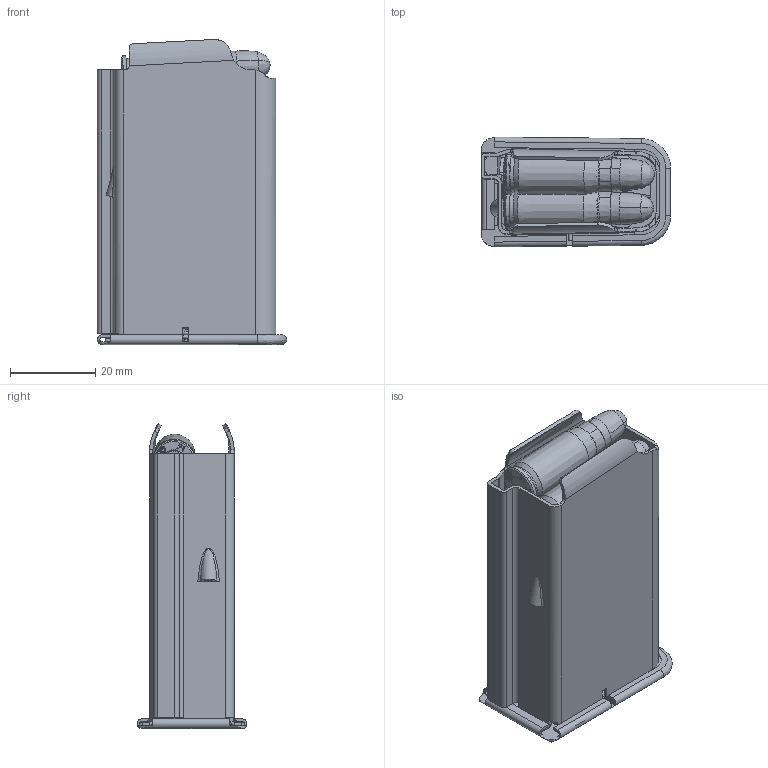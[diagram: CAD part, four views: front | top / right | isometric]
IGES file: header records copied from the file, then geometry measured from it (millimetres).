
Global section: file name: No Iges File Name specified; native system: Autodesk Inventor 2011; preprocessor: AutoDesk Inventor Iges Exporter R2011; author: EfimchenkoPA; date: 20111123.114528; units: millimetre
Bounding box: 44.5 x 25.86 x 71.75 mm (x, y, z)
Volume: 15185.1 mm3; surface area: 33232.1 mm2
Topology: 20 solids, 20 shells, 1871 faces, 4849 edges, 3076 vertices
Faces by surface type: bspline 928, plane 541, cylinder 188, revolution 122, cone 72, torus 20
